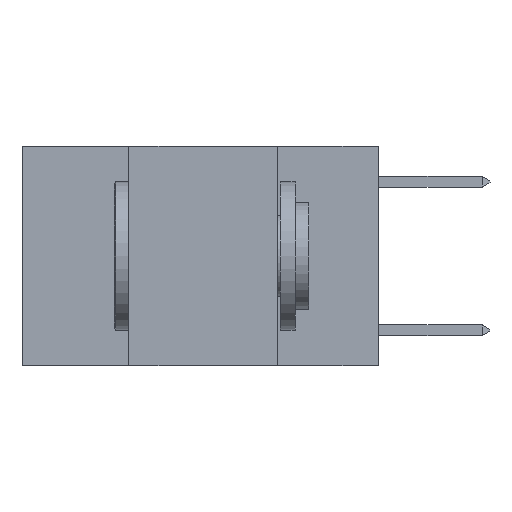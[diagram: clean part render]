
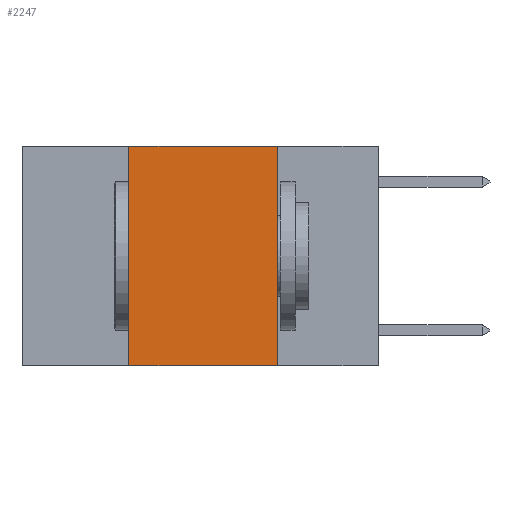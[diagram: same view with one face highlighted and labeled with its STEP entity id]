
A CAD part, left-side view. The second image highlights one B-rep face of the part: STEP entity #2247.
In plain terms, the highlighted planar face has unit normal (-1, 0, 0).
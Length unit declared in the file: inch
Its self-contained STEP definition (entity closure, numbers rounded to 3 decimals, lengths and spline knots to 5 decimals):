
#968 = PLANE ( 'NONE',  #4773 ) ;
#1006 = CARTESIAN_POINT ( 'NONE',  ( 0., 0.17, 0. ) ) ;
#1322 = CARTESIAN_POINT ( 'NONE',  ( 0., 0.42, 0. ) ) ;
#1875 = CARTESIAN_POINT ( 'NONE',  ( 0., 0.6, 0. ) ) ;
#1920 = DIRECTION ( 'NONE',  ( 1., 0., 0. ) ) ;
#1956 = LINE ( 'NONE', #1006, #4004 ) ;
#2051 = VERTEX_POINT ( 'NONE', #4139 ) ;
#2212 = VECTOR ( 'NONE', #3596, 39.37008 ) ;
#2247 = ADVANCED_FACE ( 'NONE', ( #4149 ), #968, .F. ) ;
#2370 = ORIENTED_EDGE ( 'NONE', *, *, #5159, .F. ) ;
#2578 = CARTESIAN_POINT ( 'NONE',  ( 0., 0.17, -0.37 ) ) ;
#2616 = CARTESIAN_POINT ( 'NONE',  ( 0., 0.6, 0. ) ) ;
#3023 = VECTOR ( 'NONE', #10311, 39.37008 ) ;
#3482 = LINE ( 'NONE', #6685, #10010 ) ;
#3596 = DIRECTION ( 'NONE',  ( 0., -1., 0. ) ) ;
#4004 = VECTOR ( 'NONE', #8865, 39.37008 ) ;
#4139 = CARTESIAN_POINT ( 'NONE',  ( 0., 0.17, 0. ) ) ;
#4149 = FACE_OUTER_BOUND ( 'NONE', #8573, .T. ) ;
#4462 = EDGE_CURVE ( 'NONE', #6714, #7220, #6810, .T. ) ;
#4727 = ORIENTED_EDGE ( 'NONE', *, *, #4462, .T. ) ;
#4773 = AXIS2_PLACEMENT_3D ( 'NONE', #1875, #1920, #8011 ) ;
#5159 = EDGE_CURVE ( 'NONE', #10753, #2051, #5323, .T. ) ;
#5323 = LINE ( 'NONE', #2616, #3023 ) ;
#6685 = CARTESIAN_POINT ( 'NONE',  ( 0., 0.42, 0. ) ) ;
#6714 = VERTEX_POINT ( 'NONE', #7112 ) ;
#6810 = LINE ( 'NONE', #8747, #2212 ) ;
#7112 = CARTESIAN_POINT ( 'NONE',  ( 0., 0.42, -0.37 ) ) ;
#7220 = VERTEX_POINT ( 'NONE', #2578 ) ;
#7795 = ORIENTED_EDGE ( 'NONE', *, *, #9374, .F. ) ;
#8011 = DIRECTION ( 'NONE',  ( 0., 0., -1. ) ) ;
#8573 = EDGE_LOOP ( 'NONE', ( #8816, #2370, #7795, #4727 ) ) ;
#8747 = CARTESIAN_POINT ( 'NONE',  ( 0., 0.6, -0.37 ) ) ;
#8816 = ORIENTED_EDGE ( 'NONE', *, *, #9761, .F. ) ;
#8865 = DIRECTION ( 'NONE',  ( 0., 0., -1. ) ) ;
#9374 = EDGE_CURVE ( 'NONE', #6714, #10753, #3482, .T. ) ;
#9761 = EDGE_CURVE ( 'NONE', #2051, #7220, #1956, .T. ) ;
#10010 = VECTOR ( 'NONE', #10862, 39.37008 ) ;
#10311 = DIRECTION ( 'NONE',  ( 0., -1., 0. ) ) ;
#10753 = VERTEX_POINT ( 'NONE', #1322 ) ;
#10862 = DIRECTION ( 'NONE',  ( 0., 0., 1. ) ) ;
